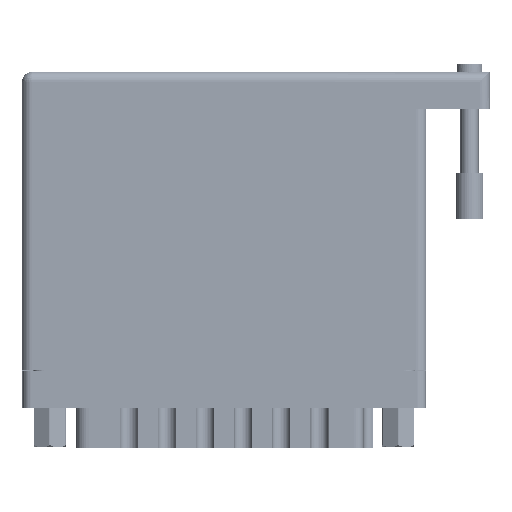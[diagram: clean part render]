
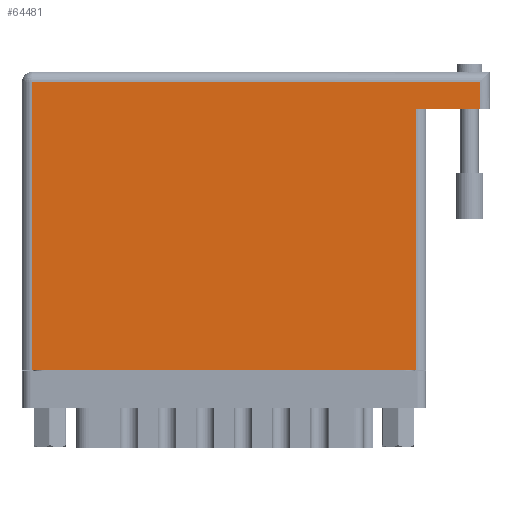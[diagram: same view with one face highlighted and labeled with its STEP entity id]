
A CAD part, front view. The second image highlights one B-rep face of the part: STEP entity #64481.
In plain terms, the highlighted face is planar.
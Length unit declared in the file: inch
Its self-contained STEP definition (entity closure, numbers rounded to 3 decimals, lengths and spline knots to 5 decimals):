
#5386 = AXIS2_PLACEMENT_3D ( 'NONE', #31944, #82331, #39971 ) ;
#7565 = EDGE_CURVE ( 'NONE', #54422, #22117, #75590, .T. ) ;
#8697 = CARTESIAN_POINT ( 'NONE',  ( 0., 1.96, 0. ) ) ;
#10455 = ORIENTED_EDGE ( 'NONE', *, *, #37740, .T. ) ;
#11207 = DIRECTION ( 'NONE',  ( -1., 0., 0. ) ) ;
#13893 = DIRECTION ( 'NONE',  ( 0., 1., 0. ) ) ;
#15981 = ORIENTED_EDGE ( 'NONE', *, *, #95074, .T. ) ;
#22117 = VERTEX_POINT ( 'NONE', #41211 ) ;
#22508 = CARTESIAN_POINT ( 'NONE',  ( 0.07, 0., 0. ) ) ;
#26274 = CARTESIAN_POINT ( 'NONE',  ( 0., 0., 0. ) ) ;
#26857 = CARTESIAN_POINT ( 'NONE',  ( 2.685, 1.774, 0. ) ) ;
#27295 = VERTEX_POINT ( 'NONE', #50361 ) ;
#30355 = FACE_OUTER_BOUND ( 'NONE', #60756, .T. ) ;
#30946 = CARTESIAN_POINT ( 'NONE',  ( 2.685, 1.774, 0. ) ) ;
#31483 = LINE ( 'NONE', #30946, #46128 ) ;
#31944 = CARTESIAN_POINT ( 'NONE',  ( 0., 2.03, 0. ) ) ;
#32527 = DIRECTION ( 'NONE',  ( 0., 1., 0. ) ) ;
#37740 = EDGE_CURVE ( 'NONE', #22117, #58352, #31483, .T. ) ;
#38339 = CARTESIAN_POINT ( 'NONE',  ( 3.19, 1.774, 0. ) ) ;
#38476 = VECTOR ( 'NONE', #64886, 39.37008 ) ;
#39971 = DIRECTION ( 'NONE',  ( -1., 0., 0. ) ) ;
#40813 = VERTEX_POINT ( 'NONE', #54405 ) ;
#40842 = DIRECTION ( 'NONE',  ( -1., 0., 0. ) ) ;
#41211 = CARTESIAN_POINT ( 'NONE',  ( 2.685, 0., 0. ) ) ;
#41863 = VECTOR ( 'NONE', #11207, 39.37008 ) ;
#46128 = VECTOR ( 'NONE', #32527, 39.37008 ) ;
#49556 = EDGE_CURVE ( 'NONE', #90986, #27295, #92703, .T. ) ;
#50361 = CARTESIAN_POINT ( 'NONE',  ( 0.07, 1.96, 0. ) ) ;
#52213 = ORIENTED_EDGE ( 'NONE', *, *, #7565, .T. ) ;
#54405 = CARTESIAN_POINT ( 'NONE',  ( 3.12, 1.774, 0. ) ) ;
#54422 = VERTEX_POINT ( 'NONE', #22508 ) ;
#54617 = LINE ( 'NONE', #77721, #92843 ) ;
#55947 = CARTESIAN_POINT ( 'NONE',  ( 0.07, 0., 0. ) ) ;
#57712 = VECTOR ( 'NONE', #40842, 39.37008 ) ;
#58352 = VERTEX_POINT ( 'NONE', #26857 ) ;
#60756 = EDGE_LOOP ( 'NONE', ( #52213, #10455, #70014, #15981, #81586, #80303 ) ) ;
#64481 = ADVANCED_FACE ( 'NONE', ( #30355 ), #65161, .F. ) ;
#64798 = EDGE_CURVE ( 'NONE', #27295, #54422, #65559, .T. ) ;
#64886 = DIRECTION ( 'NONE',  ( 1., 0., 0. ) ) ;
#65161 = PLANE ( 'NONE',  #5386 ) ;
#65559 = LINE ( 'NONE', #55947, #99590 ) ;
#67892 = EDGE_CURVE ( 'NONE', #40813, #58352, #94683, .T. ) ;
#70014 = ORIENTED_EDGE ( 'NONE', *, *, #67892, .F. ) ;
#75590 = LINE ( 'NONE', #26274, #38476 ) ;
#77721 = CARTESIAN_POINT ( 'NONE',  ( 3.12, 2.03, 0. ) ) ;
#80303 = ORIENTED_EDGE ( 'NONE', *, *, #64798, .T. ) ;
#81273 = CARTESIAN_POINT ( 'NONE',  ( 3.12, 1.96, 0. ) ) ;
#81586 = ORIENTED_EDGE ( 'NONE', *, *, #49556, .T. ) ;
#82331 = DIRECTION ( 'NONE',  ( 0., 0., -1. ) ) ;
#82735 = DIRECTION ( 'NONE',  ( 0., -1., 0. ) ) ;
#90986 = VERTEX_POINT ( 'NONE', #81273 ) ;
#92703 = LINE ( 'NONE', #8697, #57712 ) ;
#92843 = VECTOR ( 'NONE', #13893, 39.37008 ) ;
#94683 = LINE ( 'NONE', #38339, #41863 ) ;
#95074 = EDGE_CURVE ( 'NONE', #40813, #90986, #54617, .T. ) ;
#99590 = VECTOR ( 'NONE', #82735, 39.37008 ) ;
